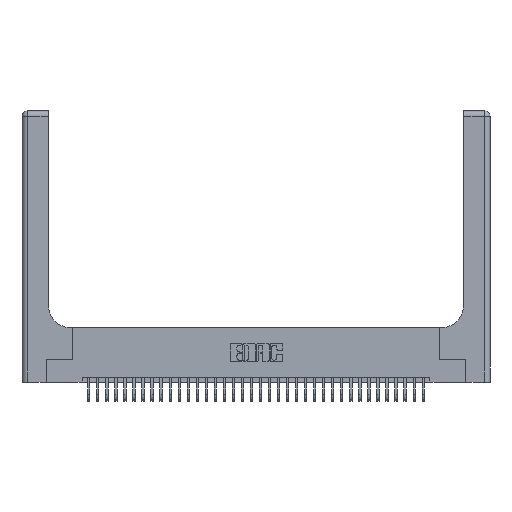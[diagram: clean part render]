
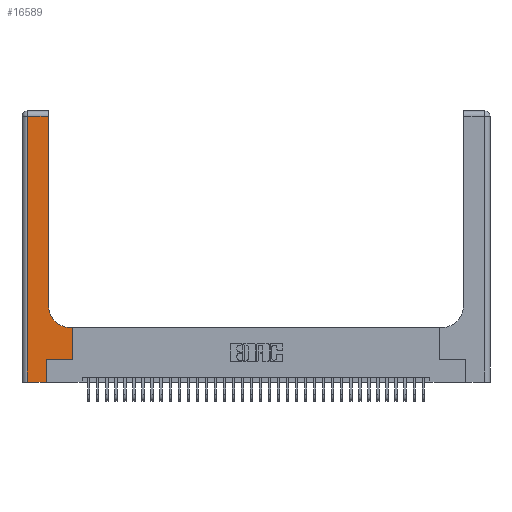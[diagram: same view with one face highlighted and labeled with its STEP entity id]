
A CAD part, top view. The second image highlights one B-rep face of the part: STEP entity #16589.
In plain terms, the highlighted planar face has unit normal (0, 0, 1).
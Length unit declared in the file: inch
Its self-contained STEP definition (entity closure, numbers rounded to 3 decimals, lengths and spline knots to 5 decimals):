
#305 = DIRECTION ( 'NONE',  ( -1., 0., 0. ) ) ;
#923 = CARTESIAN_POINT ( 'NONE',  ( 0.5415, 0.6, 0.37 ) ) ;
#1687 = VECTOR ( 'NONE', #11410, 39.37008 ) ;
#2536 = ORIENTED_EDGE ( 'NONE', *, *, #5950, .T. ) ;
#2567 = DIRECTION ( 'NONE',  ( 0., -1., 0. ) ) ;
#2839 = DIRECTION ( 'NONE',  ( 0., 0., -1. ) ) ;
#3208 = CARTESIAN_POINT ( 'NONE',  ( 0.2915, 0.6, 0.37 ) ) ;
#3572 = VECTOR ( 'NONE', #2567, 39.37008 ) ;
#3587 = VERTEX_POINT ( 'NONE', #923 ) ;
#3898 = LINE ( 'NONE', #34914, #33591 ) ;
#4121 = CARTESIAN_POINT ( 'NONE',  ( 0.2915, 3., 0.37 ) ) ;
#4424 = ORIENTED_EDGE ( 'NONE', *, *, #22626, .T. ) ;
#5057 = ORIENTED_EDGE ( 'NONE', *, *, #6103, .T. ) ;
#5927 = LINE ( 'NONE', #21744, #30124 ) ;
#5950 = EDGE_CURVE ( 'NONE', #12760, #19773, #3898, .T. ) ;
#6103 = EDGE_CURVE ( 'NONE', #8573, #7817, #29035, .T. ) ;
#6641 = LINE ( 'NONE', #4121, #34938 ) ;
#7626 = CARTESIAN_POINT ( 'NONE',  ( 0.5585, 0.25, 0.37 ) ) ;
#7817 = VERTEX_POINT ( 'NONE', #10383 ) ;
#8431 = VERTEX_POINT ( 'NONE', #37061 ) ;
#8573 = VERTEX_POINT ( 'NONE', #18155 ) ;
#8909 = FACE_OUTER_BOUND ( 'NONE', #16318, .T. ) ;
#9609 = AXIS2_PLACEMENT_3D ( 'NONE', #14620, #26464, #305 ) ;
#9863 = VERTEX_POINT ( 'NONE', #21468 ) ;
#10229 = LINE ( 'NONE', #11297, #1687 ) ;
#10383 = CARTESIAN_POINT ( 'NONE',  ( 0.06, 2.94, 0.37 ) ) ;
#11141 = CARTESIAN_POINT ( 'NONE',  ( 0.06, 3., 0.37 ) ) ;
#11297 = CARTESIAN_POINT ( 'NONE',  ( 0.269, 0., 0.37 ) ) ;
#11410 = DIRECTION ( 'NONE',  ( 0., 1., 0. ) ) ;
#12760 = VERTEX_POINT ( 'NONE', #14859 ) ;
#12793 = CARTESIAN_POINT ( 'NONE',  ( 0., 2.94, 0.37 ) ) ;
#13715 = ORIENTED_EDGE ( 'NONE', *, *, #16856, .T. ) ;
#13883 = LINE ( 'NONE', #7626, #22400 ) ;
#14426 = LINE ( 'NONE', #11141, #3572 ) ;
#14435 = CARTESIAN_POINT ( 'NONE',  ( 0.5415, 0.85, 0.37 ) ) ;
#14588 = ORIENTED_EDGE ( 'NONE', *, *, #15294, .T. ) ;
#14620 = CARTESIAN_POINT ( 'NONE',  ( 0., 3., 0.37 ) ) ;
#14859 = CARTESIAN_POINT ( 'NONE',  ( 0.06, 0., 0.37 ) ) ;
#15294 = EDGE_CURVE ( 'NONE', #35111, #9863, #5927, .T. ) ;
#15742 = EDGE_CURVE ( 'NONE', #7817, #12760, #14426, .T. ) ;
#16318 = EDGE_LOOP ( 'NONE', ( #36894, #5057, #21143, #2536, #20237, #14588, #13715, #4424, #23199 ) ) ;
#16589 = ADVANCED_FACE ( 'NONE', ( #8909 ), #26342, .F. ) ;
#16856 = EDGE_CURVE ( 'NONE', #9863, #8431, #13883, .T. ) ;
#17818 = EDGE_CURVE ( 'NONE', #19773, #35111, #10229, .T. ) ;
#18155 = CARTESIAN_POINT ( 'NONE',  ( 0.2915, 2.94, 0.37 ) ) ;
#19222 = CARTESIAN_POINT ( 'NONE',  ( 0.269, 0., 0.37 ) ) ;
#19773 = VERTEX_POINT ( 'NONE', #19222 ) ;
#19929 = DIRECTION ( 'NONE',  ( 1., 0., 0. ) ) ;
#20237 = ORIENTED_EDGE ( 'NONE', *, *, #17818, .T. ) ;
#20793 = EDGE_CURVE ( 'NONE', #3587, #33594, #31969, .T. ) ;
#21143 = ORIENTED_EDGE ( 'NONE', *, *, #15742, .T. ) ;
#21468 = CARTESIAN_POINT ( 'NONE',  ( 0.5585, 0.25, 0.37 ) ) ;
#21617 = DIRECTION ( 'NONE',  ( 1., 0., 0. ) ) ;
#21744 = CARTESIAN_POINT ( 'NONE',  ( 0.269, 0.25, 0.37 ) ) ;
#22400 = VECTOR ( 'NONE', #36365, 39.37008 ) ;
#22529 = VECTOR ( 'NONE', #35090, 39.37008 ) ;
#22626 = EDGE_CURVE ( 'NONE', #8431, #3587, #25650, .T. ) ;
#23199 = ORIENTED_EDGE ( 'NONE', *, *, #20793, .T. ) ;
#23241 = VECTOR ( 'NONE', #30612, 39.37008 ) ;
#23896 = EDGE_CURVE ( 'NONE', #33594, #8573, #6641, .T. ) ;
#25650 = LINE ( 'NONE', #3208, #22529 ) ;
#26001 = CARTESIAN_POINT ( 'NONE',  ( 0.2915, 0.85, 0.37 ) ) ;
#26342 = PLANE ( 'NONE',  #9609 ) ;
#26464 = DIRECTION ( 'NONE',  ( 0., 0., -1. ) ) ;
#28111 = DIRECTION ( 'NONE',  ( 0., 1., 0. ) ) ;
#28225 = AXIS2_PLACEMENT_3D ( 'NONE', #14435, #2839, #19929 ) ;
#29035 = LINE ( 'NONE', #12793, #23241 ) ;
#29115 = DIRECTION ( 'NONE',  ( 1., 0., 0. ) ) ;
#30124 = VECTOR ( 'NONE', #21617, 39.37008 ) ;
#30612 = DIRECTION ( 'NONE',  ( -1., 0., 0. ) ) ;
#31969 = CIRCLE ( 'NONE', #28225, 0.25 ) ;
#33591 = VECTOR ( 'NONE', #29115, 39.37008 ) ;
#33594 = VERTEX_POINT ( 'NONE', #26001 ) ;
#34914 = CARTESIAN_POINT ( 'NONE',  ( 0., 0., 0.37 ) ) ;
#34938 = VECTOR ( 'NONE', #28111, 39.37008 ) ;
#35090 = DIRECTION ( 'NONE',  ( -1., 0., 0. ) ) ;
#35111 = VERTEX_POINT ( 'NONE', #36265 ) ;
#36265 = CARTESIAN_POINT ( 'NONE',  ( 0.269, 0.25, 0.37 ) ) ;
#36365 = DIRECTION ( 'NONE',  ( 0., 1., 0. ) ) ;
#36894 = ORIENTED_EDGE ( 'NONE', *, *, #23896, .T. ) ;
#37061 = CARTESIAN_POINT ( 'NONE',  ( 0.5585, 0.6, 0.37 ) ) ;
